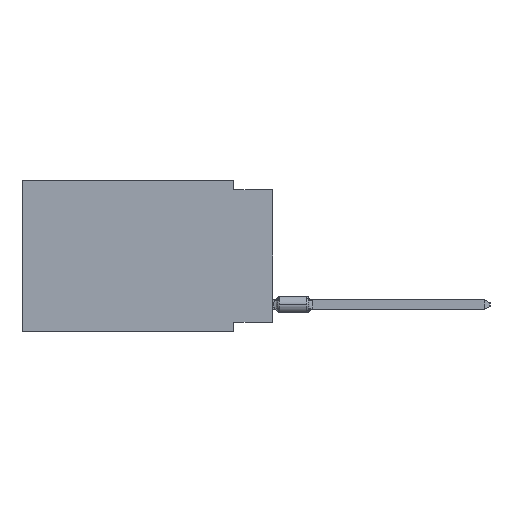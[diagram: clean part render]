
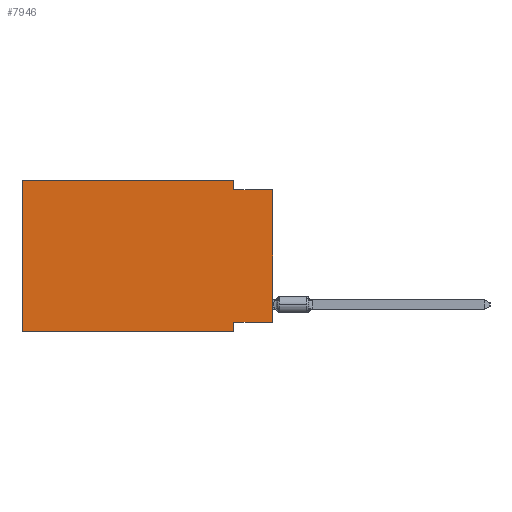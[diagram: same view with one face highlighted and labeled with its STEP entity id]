
A CAD part, left-side view. The second image highlights one B-rep face of the part: STEP entity #7946.
In plain terms, the highlighted planar face has unit normal (-1, 0, 0).
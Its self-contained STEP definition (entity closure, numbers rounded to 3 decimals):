
#134 = CARTESIAN_POINT ( 'NONE',  ( 0., 16.383, -9.906 ) ) ;
#755 = DIRECTION ( 'NONE',  ( 0., -1., 0. ) ) ;
#1153 = CARTESIAN_POINT ( 'NONE',  ( 0., 0., -0.635 ) ) ;
#2842 = VECTOR ( 'NONE', #755, 1000. ) ;
#3599 = DIRECTION ( 'NONE',  ( 0., 1., 0. ) ) ;
#3673 = DIRECTION ( 'NONE',  ( 0., -1., 0. ) ) ;
#4509 = CARTESIAN_POINT ( 'NONE',  ( 0., 2.54, 0. ) ) ;
#5384 = DIRECTION ( 'NONE',  ( 0., 0., 1. ) ) ;
#7045 = CARTESIAN_POINT ( 'NONE',  ( 0., 2.54, -9.906 ) ) ;
#7747 = ORIENTED_EDGE ( 'NONE', *, *, #30750, .T. ) ;
#7946 = ADVANCED_FACE ( 'NONE', ( #24520 ), #42862, .F. ) ;
#8950 = LINE ( 'NONE', #68259, #47676 ) ;
#9695 = EDGE_LOOP ( 'NONE', ( #50414, #37524, #66298, #11227, #16331, #7747, #16240, #58851 ) ) ;
#10217 = VECTOR ( 'NONE', #65591, 1000. ) ;
#10233 = LINE ( 'NONE', #34035, #56748 ) ;
#10301 = LINE ( 'NONE', #73917, #26211 ) ;
#11227 = ORIENTED_EDGE ( 'NONE', *, *, #74505, .F. ) ;
#14459 = EDGE_CURVE ( 'NONE', #74742, #24724, #8950, .T. ) ;
#14589 = EDGE_CURVE ( 'NONE', #35130, #23399, #23636, .T. ) ;
#14983 = VECTOR ( 'NONE', #5384, 1000. ) ;
#15730 = VERTEX_POINT ( 'NONE', #52297 ) ;
#15942 = CARTESIAN_POINT ( 'NONE',  ( 0., 2.54, 0. ) ) ;
#16240 = ORIENTED_EDGE ( 'NONE', *, *, #25108, .F. ) ;
#16331 = ORIENTED_EDGE ( 'NONE', *, *, #14459, .F. ) ;
#16549 = CARTESIAN_POINT ( 'NONE',  ( 0., 2.54, -0.635 ) ) ;
#17491 = LINE ( 'NONE', #58863, #14983 ) ;
#17766 = DIRECTION ( 'NONE',  ( 0., 0., -1. ) ) ;
#18665 = DIRECTION ( 'NONE',  ( 1., 0., 0. ) ) ;
#19945 = VERTEX_POINT ( 'NONE', #32638 ) ;
#23399 = VERTEX_POINT ( 'NONE', #16549 ) ;
#23636 = LINE ( 'NONE', #15942, #71335 ) ;
#23808 = LINE ( 'NONE', #1153, #2842 ) ;
#24520 = FACE_OUTER_BOUND ( 'NONE', #9695, .T. ) ;
#24724 = VERTEX_POINT ( 'NONE', #30186 ) ;
#25108 = EDGE_CURVE ( 'NONE', #42465, #15730, #25396, .T. ) ;
#25396 = LINE ( 'NONE', #7045, #10217 ) ;
#26142 = DIRECTION ( 'NONE',  ( 0., 0., 1. ) ) ;
#26211 = VECTOR ( 'NONE', #3673, 1000. ) ;
#29874 = AXIS2_PLACEMENT_3D ( 'NONE', #48332, #18665, #42483 ) ;
#30186 = CARTESIAN_POINT ( 'NONE',  ( 0., 16.383, 0. ) ) ;
#30750 = EDGE_CURVE ( 'NONE', #74742, #15730, #10301, .T. ) ;
#32638 = CARTESIAN_POINT ( 'NONE',  ( 0., 0., -9.271 ) ) ;
#33457 = LINE ( 'NONE', #45195, #39644 ) ;
#34035 = CARTESIAN_POINT ( 'NONE',  ( 0., 0., -9.271 ) ) ;
#35130 = VERTEX_POINT ( 'NONE', #4509 ) ;
#36439 = EDGE_CURVE ( 'NONE', #19945, #60820, #17491, .T. ) ;
#37524 = ORIENTED_EDGE ( 'NONE', *, *, #66458, .F. ) ;
#39644 = VECTOR ( 'NONE', #56876, 1000. ) ;
#42465 = VERTEX_POINT ( 'NONE', #43049 ) ;
#42483 = DIRECTION ( 'NONE',  ( 0., 0., -1. ) ) ;
#42862 = PLANE ( 'NONE',  #29874 ) ;
#43049 = CARTESIAN_POINT ( 'NONE',  ( 0., 2.54, -9.271 ) ) ;
#45195 = CARTESIAN_POINT ( 'NONE',  ( 0., 16.383, 0. ) ) ;
#47676 = VECTOR ( 'NONE', #26142, 1000. ) ;
#47800 = CARTESIAN_POINT ( 'NONE',  ( 0., 0., -0.635 ) ) ;
#48332 = CARTESIAN_POINT ( 'NONE',  ( 0., 16.383, 0. ) ) ;
#50414 = ORIENTED_EDGE ( 'NONE', *, *, #36439, .T. ) ;
#52297 = CARTESIAN_POINT ( 'NONE',  ( 0., 2.54, -9.906 ) ) ;
#55660 = EDGE_CURVE ( 'NONE', #19945, #42465, #10233, .T. ) ;
#56748 = VECTOR ( 'NONE', #3599, 1000. ) ;
#56876 = DIRECTION ( 'NONE',  ( 0., -1., 0. ) ) ;
#58851 = ORIENTED_EDGE ( 'NONE', *, *, #55660, .F. ) ;
#58863 = CARTESIAN_POINT ( 'NONE',  ( 0., 0., 0. ) ) ;
#60820 = VERTEX_POINT ( 'NONE', #47800 ) ;
#65591 = DIRECTION ( 'NONE',  ( 0., 0., -1. ) ) ;
#66298 = ORIENTED_EDGE ( 'NONE', *, *, #14589, .F. ) ;
#66458 = EDGE_CURVE ( 'NONE', #23399, #60820, #23808, .T. ) ;
#68259 = CARTESIAN_POINT ( 'NONE',  ( 0., 16.383, 0. ) ) ;
#71335 = VECTOR ( 'NONE', #17766, 1000. ) ;
#73917 = CARTESIAN_POINT ( 'NONE',  ( 0., 16.383, -9.906 ) ) ;
#74505 = EDGE_CURVE ( 'NONE', #24724, #35130, #33457, .T. ) ;
#74742 = VERTEX_POINT ( 'NONE', #134 ) ;
